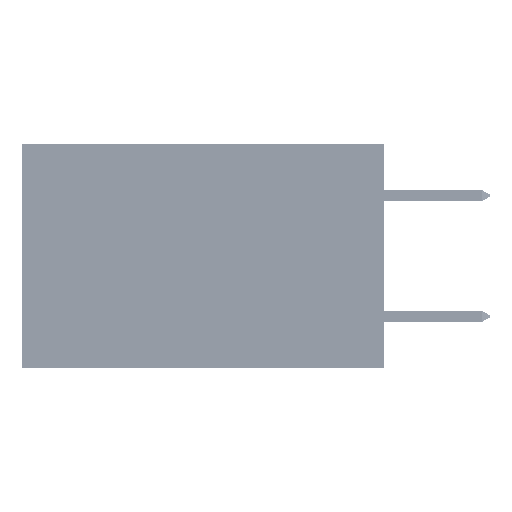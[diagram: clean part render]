
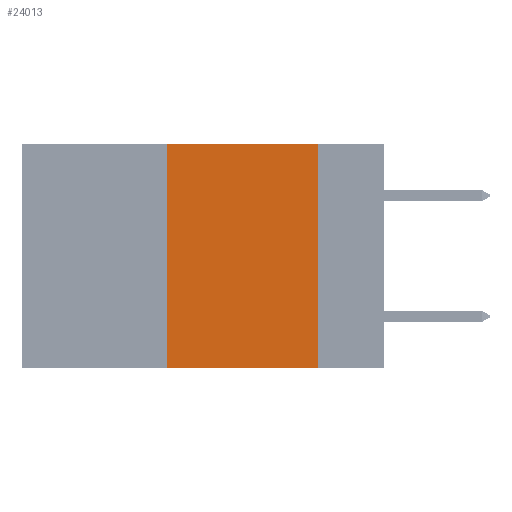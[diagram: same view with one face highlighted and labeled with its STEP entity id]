
A CAD part, left-side view. The second image highlights one B-rep face of the part: STEP entity #24013.
In plain terms, the highlighted planar face has unit normal (-1, 0, 0).
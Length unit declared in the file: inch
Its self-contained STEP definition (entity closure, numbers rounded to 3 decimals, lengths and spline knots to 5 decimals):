
#249 = CARTESIAN_POINT ( 'NONE',  ( 0., 0.36, -0.37 ) ) ;
#923 = CARTESIAN_POINT ( 'NONE',  ( 0., 0.36, 0. ) ) ;
#1562 = DIRECTION ( 'NONE',  ( 0., 0., -1. ) ) ;
#2967 = DIRECTION ( 'NONE',  ( 1., 0., 0. ) ) ;
#6881 = VECTOR ( 'NONE', #27851, 39.37008 ) ;
#7852 = VERTEX_POINT ( 'NONE', #32181 ) ;
#8503 = EDGE_CURVE ( 'NONE', #14270, #22415, #14874, .T. ) ;
#8559 = LINE ( 'NONE', #40220, #25911 ) ;
#9429 = CARTESIAN_POINT ( 'NONE',  ( 0., 0.11, 0. ) ) ;
#9947 = CARTESIAN_POINT ( 'NONE',  ( 0., 0.6, 0. ) ) ;
#10204 = VECTOR ( 'NONE', #44386, 39.37008 ) ;
#11692 = EDGE_CURVE ( 'NONE', #22415, #15697, #34604, .T. ) ;
#14270 = VERTEX_POINT ( 'NONE', #249 ) ;
#14874 = LINE ( 'NONE', #29080, #10204 ) ;
#15399 = ORIENTED_EDGE ( 'NONE', *, *, #11692, .F. ) ;
#15697 = VERTEX_POINT ( 'NONE', #9429 ) ;
#15777 = DIRECTION ( 'NONE',  ( 0., -1., 0. ) ) ;
#16238 = LINE ( 'NONE', #37194, #35186 ) ;
#16666 = CARTESIAN_POINT ( 'NONE',  ( 0., 0.6, 0. ) ) ;
#17316 = AXIS2_PLACEMENT_3D ( 'NONE', #9947, #2967, #27882 ) ;
#20116 = ORIENTED_EDGE ( 'NONE', *, *, #28823, .T. ) ;
#22415 = VERTEX_POINT ( 'NONE', #923 ) ;
#22576 = ORIENTED_EDGE ( 'NONE', *, *, #40992, .F. ) ;
#24013 = ADVANCED_FACE ( 'NONE', ( #41868 ), #31373, .F. ) ;
#25911 = VECTOR ( 'NONE', #1562, 39.37008 ) ;
#27851 = DIRECTION ( 'NONE',  ( 0., -1., 0. ) ) ;
#27882 = DIRECTION ( 'NONE',  ( 0., 0., -1. ) ) ;
#28823 = EDGE_CURVE ( 'NONE', #14270, #7852, #16238, .T. ) ;
#29080 = CARTESIAN_POINT ( 'NONE',  ( 0., 0.36, 0. ) ) ;
#31373 = PLANE ( 'NONE',  #17316 ) ;
#31628 = ORIENTED_EDGE ( 'NONE', *, *, #8503, .F. ) ;
#32181 = CARTESIAN_POINT ( 'NONE',  ( 0., 0.11, -0.37 ) ) ;
#34604 = LINE ( 'NONE', #16666, #6881 ) ;
#35186 = VECTOR ( 'NONE', #15777, 39.37008 ) ;
#37194 = CARTESIAN_POINT ( 'NONE',  ( 0., 0.6, -0.37 ) ) ;
#37750 = EDGE_LOOP ( 'NONE', ( #22576, #15399, #31628, #20116 ) ) ;
#40220 = CARTESIAN_POINT ( 'NONE',  ( 0., 0.11, 0. ) ) ;
#40992 = EDGE_CURVE ( 'NONE', #15697, #7852, #8559, .T. ) ;
#41868 = FACE_OUTER_BOUND ( 'NONE', #37750, .T. ) ;
#44386 = DIRECTION ( 'NONE',  ( 0., 0., 1. ) ) ;
